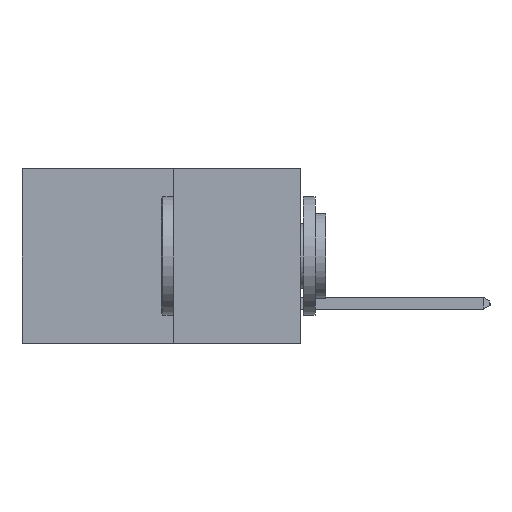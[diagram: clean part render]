
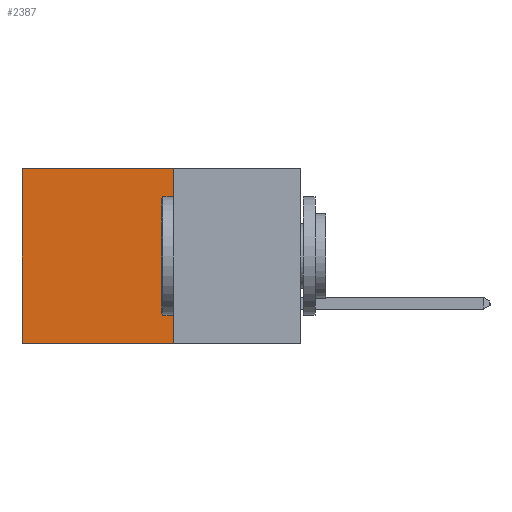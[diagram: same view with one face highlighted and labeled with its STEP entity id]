
A CAD part, left-side view. The second image highlights one B-rep face of the part: STEP entity #2387.
In plain terms, the highlighted planar face has unit normal (-1, 0, 0).
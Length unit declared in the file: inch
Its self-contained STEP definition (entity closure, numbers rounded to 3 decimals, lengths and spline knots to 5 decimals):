
#534 = CARTESIAN_POINT ( 'NONE',  ( 0.277, 0.27, -0.37 ) ) ;
#703 = EDGE_LOOP ( 'NONE', ( #9328, #4472, #12501, #7672 ) ) ;
#717 = CARTESIAN_POINT ( 'NONE',  ( 0.277, 0.59, 0. ) ) ;
#743 = DIRECTION ( 'NONE',  ( 0., 0., -1. ) ) ;
#1066 = VECTOR ( 'NONE', #3699, 39.37008 ) ;
#1252 = CARTESIAN_POINT ( 'NONE',  ( 0.277, 0.59, -0.37 ) ) ;
#1357 = AXIS2_PLACEMENT_3D ( 'NONE', #4239, #5882, #2765 ) ;
#1388 = LINE ( 'NONE', #4629, #1066 ) ;
#1563 = DIRECTION ( 'NONE',  ( 0., 1., 0. ) ) ;
#1976 = LINE ( 'NONE', #11591, #9544 ) ;
#2387 = ADVANCED_FACE ( 'NONE', ( #5819 ), #5102, .F. ) ;
#2765 = DIRECTION ( 'NONE',  ( 0., 0., -1. ) ) ;
#3008 = CARTESIAN_POINT ( 'NONE',  ( 0.277, 0.59, -0.37 ) ) ;
#3310 = CARTESIAN_POINT ( 'NONE',  ( 0.277, 0.27, -0.37 ) ) ;
#3699 = DIRECTION ( 'NONE',  ( 0., 1., 0. ) ) ;
#4027 = VERTEX_POINT ( 'NONE', #717 ) ;
#4239 = CARTESIAN_POINT ( 'NONE',  ( 0.277, 0.27, -0.37 ) ) ;
#4389 = VERTEX_POINT ( 'NONE', #11070 ) ;
#4472 = ORIENTED_EDGE ( 'NONE', *, *, #8355, .F. ) ;
#4629 = CARTESIAN_POINT ( 'NONE',  ( 0.277, 0.27, 0. ) ) ;
#5102 = PLANE ( 'NONE',  #1357 ) ;
#5819 = FACE_OUTER_BOUND ( 'NONE', #703, .T. ) ;
#5882 = DIRECTION ( 'NONE',  ( 1., 0., 0. ) ) ;
#6934 = EDGE_CURVE ( 'NONE', #4389, #4027, #1388, .T. ) ;
#7408 = LINE ( 'NONE', #534, #12261 ) ;
#7672 = ORIENTED_EDGE ( 'NONE', *, *, #6934, .T. ) ;
#8355 = EDGE_CURVE ( 'NONE', #11201, #8663, #7408, .T. ) ;
#8663 = VERTEX_POINT ( 'NONE', #3008 ) ;
#8791 = EDGE_CURVE ( 'NONE', #4027, #8663, #10373, .T. ) ;
#9328 = ORIENTED_EDGE ( 'NONE', *, *, #8791, .T. ) ;
#9544 = VECTOR ( 'NONE', #743, 39.37008 ) ;
#10373 = LINE ( 'NONE', #1252, #12606 ) ;
#10853 = EDGE_CURVE ( 'NONE', #4389, #11201, #1976, .T. ) ;
#11070 = CARTESIAN_POINT ( 'NONE',  ( 0.277, 0.27, 0. ) ) ;
#11201 = VERTEX_POINT ( 'NONE', #3310 ) ;
#11591 = CARTESIAN_POINT ( 'NONE',  ( 0.277, 0.27, -0.37 ) ) ;
#12052 = DIRECTION ( 'NONE',  ( 0., 0., -1. ) ) ;
#12261 = VECTOR ( 'NONE', #1563, 39.37008 ) ;
#12501 = ORIENTED_EDGE ( 'NONE', *, *, #10853, .F. ) ;
#12606 = VECTOR ( 'NONE', #12052, 39.37008 ) ;
